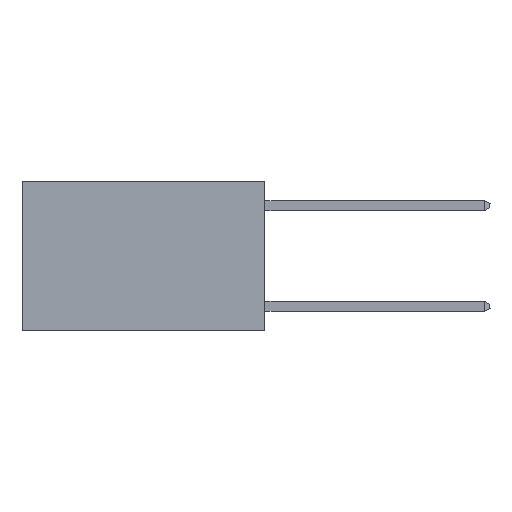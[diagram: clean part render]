
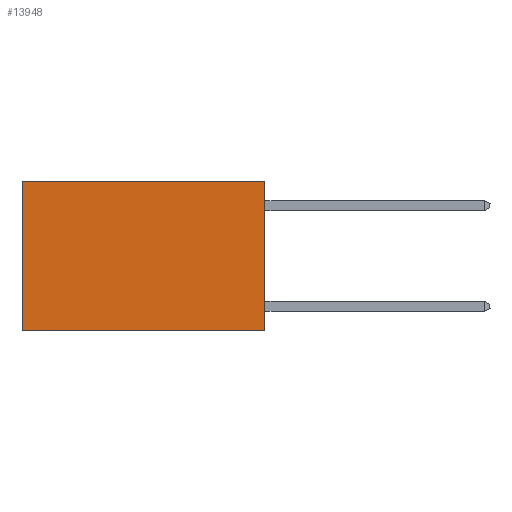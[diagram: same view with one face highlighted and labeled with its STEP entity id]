
A CAD part, left-side view. The second image highlights one B-rep face of the part: STEP entity #13948.
In plain terms, the highlighted planar face has unit normal (-1, 0, 0).
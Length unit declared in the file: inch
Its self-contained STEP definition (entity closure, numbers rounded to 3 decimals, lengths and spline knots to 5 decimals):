
#222 = VECTOR ( 'NONE', #19695, 39.37008 ) ;
#474 = VERTEX_POINT ( 'NONE', #13357 ) ;
#898 = CARTESIAN_POINT ( 'NONE',  ( 0.2625, 0., 0. ) ) ;
#1256 = VERTEX_POINT ( 'NONE', #14697 ) ;
#1267 = EDGE_CURVE ( 'NONE', #474, #1256, #19799, .T. ) ;
#1888 = CARTESIAN_POINT ( 'NONE',  ( 0.2625, 0., -0.37 ) ) ;
#1961 = AXIS2_PLACEMENT_3D ( 'NONE', #7599, #2811, #21091 ) ;
#2811 = DIRECTION ( 'NONE',  ( 1., 0., 0. ) ) ;
#3660 = ORIENTED_EDGE ( 'NONE', *, *, #1267, .T. ) ;
#3690 = VECTOR ( 'NONE', #18168, 39.37008 ) ;
#3960 = LINE ( 'NONE', #10251, #7446 ) ;
#4177 = ORIENTED_EDGE ( 'NONE', *, *, #11208, .T. ) ;
#4906 = CARTESIAN_POINT ( 'NONE',  ( 0.2625, 0.6, 0. ) ) ;
#4918 = LINE ( 'NONE', #18015, #12280 ) ;
#5026 = DIRECTION ( 'NONE',  ( 0., 0., -1. ) ) ;
#7446 = VECTOR ( 'NONE', #16892, 39.37008 ) ;
#7464 = EDGE_LOOP ( 'NONE', ( #3660, #11058, #18381, #4177 ) ) ;
#7599 = CARTESIAN_POINT ( 'NONE',  ( 0.2625, 0., 0. ) ) ;
#9217 = FACE_OUTER_BOUND ( 'NONE', #7464, .T. ) ;
#10251 = CARTESIAN_POINT ( 'NONE',  ( 0.2625, 0., 0. ) ) ;
#11011 = CARTESIAN_POINT ( 'NONE',  ( 0.2625, 0., -0.37 ) ) ;
#11058 = ORIENTED_EDGE ( 'NONE', *, *, #18487, .F. ) ;
#11208 = EDGE_CURVE ( 'NONE', #18675, #474, #3960, .T. ) ;
#12280 = VECTOR ( 'NONE', #5026, 39.37008 ) ;
#13357 = CARTESIAN_POINT ( 'NONE',  ( 0.2625, 0.6, 0. ) ) ;
#13948 = ADVANCED_FACE ( 'NONE', ( #9217 ), #20874, .F. ) ;
#14697 = CARTESIAN_POINT ( 'NONE',  ( 0.2625, 0.6, -0.37 ) ) ;
#16057 = VERTEX_POINT ( 'NONE', #11011 ) ;
#16242 = EDGE_CURVE ( 'NONE', #18675, #16057, #4918, .T. ) ;
#16663 = LINE ( 'NONE', #1888, #3690 ) ;
#16892 = DIRECTION ( 'NONE',  ( 0., 1., 0. ) ) ;
#18015 = CARTESIAN_POINT ( 'NONE',  ( 0.2625, 0., 0. ) ) ;
#18168 = DIRECTION ( 'NONE',  ( 0., 1., 0. ) ) ;
#18381 = ORIENTED_EDGE ( 'NONE', *, *, #16242, .F. ) ;
#18487 = EDGE_CURVE ( 'NONE', #16057, #1256, #16663, .T. ) ;
#18675 = VERTEX_POINT ( 'NONE', #898 ) ;
#19695 = DIRECTION ( 'NONE',  ( 0., 0., -1. ) ) ;
#19799 = LINE ( 'NONE', #4906, #222 ) ;
#20874 = PLANE ( 'NONE',  #1961 ) ;
#21091 = DIRECTION ( 'NONE',  ( 0., 0., -1. ) ) ;
